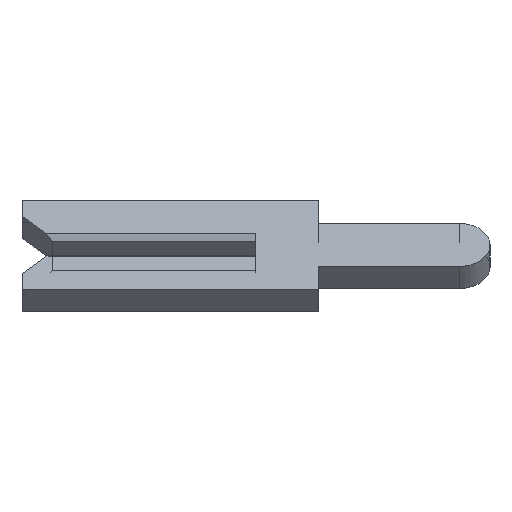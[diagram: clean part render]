
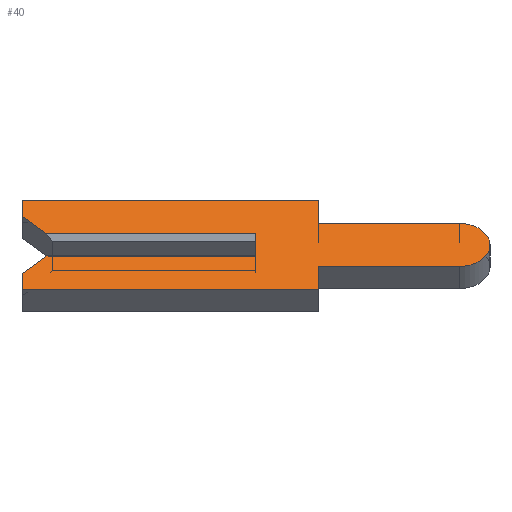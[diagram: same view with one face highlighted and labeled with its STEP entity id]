
A CAD part, left-side view. The second image highlights one B-rep face of the part: STEP entity #40.
In plain terms, the highlighted face is planar.
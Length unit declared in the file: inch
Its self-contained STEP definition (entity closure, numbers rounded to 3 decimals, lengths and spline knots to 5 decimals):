
#8 = CARTESIAN_POINT ( 'NONE',  ( -0.01, 0., 0.0065 ) ) ;
#19 = DIRECTION ( 'NONE',  ( 0., -1., 0. ) ) ;
#24 = LINE ( 'NONE', #1748, #1490 ) ;
#29 = VERTEX_POINT ( 'NONE', #791 ) ;
#40 = ADVANCED_FACE ( 'NONE', ( #2109 ), #1211, .F. ) ;
#45 = DIRECTION ( 'NONE',  ( 1., 0., 0. ) ) ;
#83 = LINE ( 'NONE', #2791, #2367 ) ;
#95 = VERTEX_POINT ( 'NONE', #2350 ) ;
#113 = EDGE_CURVE ( 'NONE', #1638, #750, #837, .T. ) ;
#125 = CARTESIAN_POINT ( 'NONE',  ( -0.01, -0.04, -0.0195 ) ) ;
#158 = ORIENTED_EDGE ( 'NONE', *, *, #2388, .F. ) ;
#166 = VERTEX_POINT ( 'NONE', #1012 ) ;
#183 = CARTESIAN_POINT ( 'NONE',  ( -0.01, 0.134, -0.01 ) ) ;
#185 = VECTOR ( 'NONE', #2162, 39.37008 ) ;
#207 = DIRECTION ( 'NONE',  ( 0., 0.707, 0.707 ) ) ;
#237 = CARTESIAN_POINT ( 'NONE',  ( -0.01, -0.1305, -0.01 ) ) ;
#274 = ORIENTED_EDGE ( 'NONE', *, *, #1323, .F. ) ;
#307 = EDGE_CURVE ( 'NONE', #1601, #1099, #2254, .T. ) ;
#459 = DIRECTION ( 'NONE',  ( 0., 1., 0. ) ) ;
#491 = CARTESIAN_POINT ( 'NONE',  ( -0.01, -0.04, 0.0195 ) ) ;
#503 = VERTEX_POINT ( 'NONE', #1059 ) ;
#557 = DIRECTION ( 'NONE',  ( 0., -1., 0. ) ) ;
#583 = ORIENTED_EDGE ( 'NONE', *, *, #2520, .F. ) ;
#608 = CARTESIAN_POINT ( 'NONE',  ( -0.01, 0.15, -0.04 ) ) ;
#668 = EDGE_CURVE ( 'NONE', #1533, #1099, #2291, .T. ) ;
#679 = CARTESIAN_POINT ( 'NONE',  ( -0.01, 0.15, 0.01 ) ) ;
#710 = DIRECTION ( 'NONE',  ( 0., 0., -1. ) ) ;
#729 = EDGE_CURVE ( 'NONE', #750, #1533, #2360, .T. ) ;
#750 = VERTEX_POINT ( 'NONE', #183 ) ;
#753 = EDGE_CURVE ( 'NONE', #1387, #1541, #1165, .T. ) ;
#777 = DIRECTION ( 'NONE',  ( 0., 1., 0. ) ) ;
#791 = CARTESIAN_POINT ( 'NONE',  ( -0.01, -0.04, 0.0195 ) ) ;
#833 = DIRECTION ( 'NONE',  ( 1., 0., 0. ) ) ;
#837 = LINE ( 'NONE', #2587, #2518 ) ;
#873 = CARTESIAN_POINT ( 'NONE',  ( -0.01, 0.15, 0.026 ) ) ;
#897 = CARTESIAN_POINT ( 'NONE',  ( -0.01, -0.04, -0.0195 ) ) ;
#1012 = CARTESIAN_POINT ( 'NONE',  ( -0.01, -0.04, 0.04 ) ) ;
#1024 = ORIENTED_EDGE ( 'NONE', *, *, #1905, .F. ) ;
#1059 = CARTESIAN_POINT ( 'NONE',  ( -0.01, -0.1305, 0.0195 ) ) ;
#1097 = VECTOR ( 'NONE', #459, 39.37008 ) ;
#1099 = VERTEX_POINT ( 'NONE', #2023 ) ;
#1153 = CARTESIAN_POINT ( 'NONE',  ( -0.01, -0.04, 0.04 ) ) ;
#1165 = LINE ( 'NONE', #897, #1097 ) ;
#1211 = PLANE ( 'NONE',  #1510 ) ;
#1230 = CARTESIAN_POINT ( 'NONE',  ( -0.01, -0.1305, 0. ) ) ;
#1262 = DIRECTION ( 'NONE',  ( 0., -0.707, 0.707 ) ) ;
#1266 = CARTESIAN_POINT ( 'NONE',  ( -0.01, 0.134, 0.01 ) ) ;
#1285 = VERTEX_POINT ( 'NONE', #1384 ) ;
#1305 = EDGE_CURVE ( 'NONE', #503, #1387, #1531, .T. ) ;
#1323 = EDGE_CURVE ( 'NONE', #29, #503, #1898, .T. ) ;
#1384 = CARTESIAN_POINT ( 'NONE',  ( -0.01, 0.15, 0.04 ) ) ;
#1387 = VERTEX_POINT ( 'NONE', #2466 ) ;
#1410 = EDGE_CURVE ( 'NONE', #166, #29, #1693, .T. ) ;
#1438 = DIRECTION ( 'NONE',  ( 0., 0., -1. ) ) ;
#1458 = VECTOR ( 'NONE', #2681, 39.37008 ) ;
#1490 = VECTOR ( 'NONE', #207, 39.37008 ) ;
#1510 = AXIS2_PLACEMENT_3D ( 'NONE', #1230, #833, #1925 ) ;
#1516 = DIRECTION ( 'NONE',  ( 0., 0., -1. ) ) ;
#1531 = CIRCLE ( 'NONE', #1570, 0.0195 ) ;
#1533 = VERTEX_POINT ( 'NONE', #2239 ) ;
#1541 = VERTEX_POINT ( 'NONE', #125 ) ;
#1570 = AXIS2_PLACEMENT_3D ( 'NONE', #1812, #45, #710 ) ;
#1601 = VERTEX_POINT ( 'NONE', #1266 ) ;
#1629 = VECTOR ( 'NONE', #1438, 39.37008 ) ;
#1638 = VERTEX_POINT ( 'NONE', #2534 ) ;
#1678 = DIRECTION ( 'NONE',  ( 0., -1., 0. ) ) ;
#1693 = LINE ( 'NONE', #1153, #1629 ) ;
#1701 = EDGE_LOOP ( 'NONE', ( #2813, #2808, #2580, #1900, #1024, #2733, #158, #2180, #2248, #274, #2628, #2016, #2721, #583 ) ) ;
#1748 = CARTESIAN_POINT ( 'NONE',  ( -0.01, 0.1305, 0.0065 ) ) ;
#1784 = VECTOR ( 'NONE', #2389, 39.37008 ) ;
#1812 = CARTESIAN_POINT ( 'NONE',  ( -0.01, -0.1305, 0. ) ) ;
#1898 = LINE ( 'NONE', #491, #2503 ) ;
#1900 = ORIENTED_EDGE ( 'NONE', *, *, #113, .F. ) ;
#1905 = EDGE_CURVE ( 'NONE', #95, #1638, #2034, .T. ) ;
#1920 = CARTESIAN_POINT ( 'NONE',  ( -0.01, -0.04, -0.04 ) ) ;
#1925 = DIRECTION ( 'NONE',  ( 0., 0., -1. ) ) ;
#1998 = VERTEX_POINT ( 'NONE', #2780 ) ;
#2000 = EDGE_CURVE ( 'NONE', #2138, #95, #2525, .T. ) ;
#2008 = CARTESIAN_POINT ( 'NONE',  ( -0.01, -0.04, -0.04 ) ) ;
#2016 = ORIENTED_EDGE ( 'NONE', *, *, #2046, .F. ) ;
#2023 = CARTESIAN_POINT ( 'NONE',  ( -0.01, 0., 0.01 ) ) ;
#2034 = LINE ( 'NONE', #2207, #1458 ) ;
#2046 = EDGE_CURVE ( 'NONE', #1285, #166, #83, .T. ) ;
#2109 = FACE_OUTER_BOUND ( 'NONE', #1701, .T. ) ;
#2138 = VERTEX_POINT ( 'NONE', #1920 ) ;
#2162 = DIRECTION ( 'NONE',  ( 0., 0., 1. ) ) ;
#2178 = VECTOR ( 'NONE', #2664, 39.37008 ) ;
#2180 = ORIENTED_EDGE ( 'NONE', *, *, #753, .F. ) ;
#2186 = VECTOR ( 'NONE', #19, 39.37008 ) ;
#2207 = CARTESIAN_POINT ( 'NONE',  ( -0.01, 0.15, -0.026 ) ) ;
#2239 = CARTESIAN_POINT ( 'NONE',  ( -0.01, 0., -0.01 ) ) ;
#2248 = ORIENTED_EDGE ( 'NONE', *, *, #1305, .F. ) ;
#2254 = LINE ( 'NONE', #679, #2186 ) ;
#2291 = LINE ( 'NONE', #8, #185 ) ;
#2350 = CARTESIAN_POINT ( 'NONE',  ( -0.01, 0.15, -0.04 ) ) ;
#2360 = LINE ( 'NONE', #237, #1784 ) ;
#2367 = VECTOR ( 'NONE', #1678, 39.37008 ) ;
#2388 = EDGE_CURVE ( 'NONE', #1541, #2138, #2717, .T. ) ;
#2389 = DIRECTION ( 'NONE',  ( 0., -1., 0. ) ) ;
#2456 = VECTOR ( 'NONE', #777, 39.37008 ) ;
#2466 = CARTESIAN_POINT ( 'NONE',  ( -0.01, -0.1305, -0.0195 ) ) ;
#2476 = LINE ( 'NONE', #873, #2178 ) ;
#2503 = VECTOR ( 'NONE', #557, 39.37008 ) ;
#2518 = VECTOR ( 'NONE', #1262, 39.37008 ) ;
#2520 = EDGE_CURVE ( 'NONE', #1601, #1998, #24, .T. ) ;
#2525 = LINE ( 'NONE', #608, #2456 ) ;
#2534 = CARTESIAN_POINT ( 'NONE',  ( -0.01, 0.15, -0.026 ) ) ;
#2580 = ORIENTED_EDGE ( 'NONE', *, *, #729, .F. ) ;
#2587 = CARTESIAN_POINT ( 'NONE',  ( -0.01, 0.1305, -0.0065 ) ) ;
#2619 = VECTOR ( 'NONE', #1516, 39.37008 ) ;
#2628 = ORIENTED_EDGE ( 'NONE', *, *, #1410, .F. ) ;
#2664 = DIRECTION ( 'NONE',  ( 0., 0., 1. ) ) ;
#2681 = DIRECTION ( 'NONE',  ( 0., 0., 1. ) ) ;
#2717 = LINE ( 'NONE', #2008, #2619 ) ;
#2721 = ORIENTED_EDGE ( 'NONE', *, *, #2764, .F. ) ;
#2733 = ORIENTED_EDGE ( 'NONE', *, *, #2000, .F. ) ;
#2764 = EDGE_CURVE ( 'NONE', #1998, #1285, #2476, .T. ) ;
#2780 = CARTESIAN_POINT ( 'NONE',  ( -0.01, 0.15, 0.026 ) ) ;
#2791 = CARTESIAN_POINT ( 'NONE',  ( -0.01, 0.15, 0.04 ) ) ;
#2808 = ORIENTED_EDGE ( 'NONE', *, *, #668, .F. ) ;
#2813 = ORIENTED_EDGE ( 'NONE', *, *, #307, .T. ) ;
